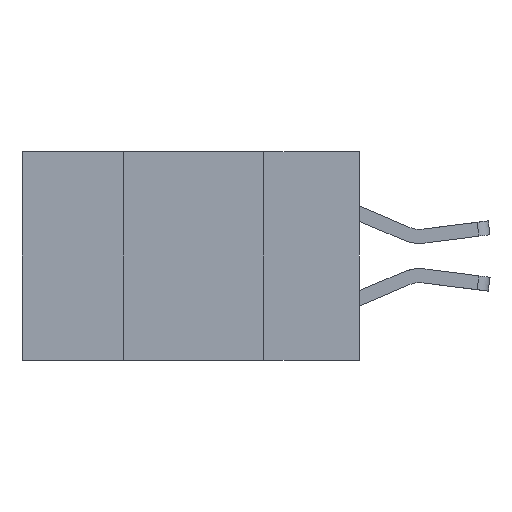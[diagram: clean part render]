
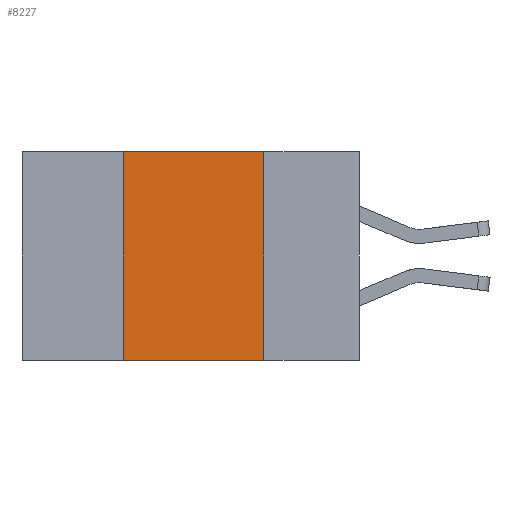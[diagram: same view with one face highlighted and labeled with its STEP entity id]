
A CAD part, left-side view. The second image highlights one B-rep face of the part: STEP entity #8227.
In plain terms, the highlighted planar face has unit normal (-1, 0, 0).
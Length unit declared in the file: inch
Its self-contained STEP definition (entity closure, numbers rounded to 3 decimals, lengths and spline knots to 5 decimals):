
#322 = LINE ( 'NONE', #11285, #13286 ) ;
#830 = LINE ( 'NONE', #6893, #8939 ) ;
#1108 = VERTEX_POINT ( 'NONE', #7104 ) ;
#1424 = DIRECTION ( 'NONE',  ( 0., 0., 1. ) ) ;
#1754 = CARTESIAN_POINT ( 'NONE',  ( 0., 0.17, 0. ) ) ;
#2039 = VECTOR ( 'NONE', #1424, 39.37008 ) ;
#2238 = PLANE ( 'NONE',  #13112 ) ;
#2888 = EDGE_CURVE ( 'NONE', #1108, #5336, #322, .T. ) ;
#3066 = EDGE_CURVE ( 'NONE', #7118, #10564, #830, .T. ) ;
#3133 = FACE_OUTER_BOUND ( 'NONE', #12243, .T. ) ;
#4411 = CARTESIAN_POINT ( 'NONE',  ( 0., 0.6, 0. ) ) ;
#4841 = EDGE_CURVE ( 'NONE', #7118, #1108, #7668, .T. ) ;
#5336 = VERTEX_POINT ( 'NONE', #9639 ) ;
#5516 = DIRECTION ( 'NONE',  ( 1., 0., 0. ) ) ;
#6893 = CARTESIAN_POINT ( 'NONE',  ( 0., 0.6, -0.37 ) ) ;
#6995 = DIRECTION ( 'NONE',  ( 0., -1., 0. ) ) ;
#7104 = CARTESIAN_POINT ( 'NONE',  ( 0., 0.42, 0. ) ) ;
#7118 = VERTEX_POINT ( 'NONE', #11430 ) ;
#7126 = DIRECTION ( 'NONE',  ( 0., 0., -1. ) ) ;
#7580 = LINE ( 'NONE', #1754, #12492 ) ;
#7668 = LINE ( 'NONE', #8759, #2039 ) ;
#8227 = ADVANCED_FACE ( 'NONE', ( #3133 ), #2238, .F. ) ;
#8576 = EDGE_CURVE ( 'NONE', #5336, #10564, #7580, .T. ) ;
#8759 = CARTESIAN_POINT ( 'NONE',  ( 0., 0.42, 0. ) ) ;
#8939 = VECTOR ( 'NONE', #6995, 39.37008 ) ;
#9639 = CARTESIAN_POINT ( 'NONE',  ( 0., 0.17, 0. ) ) ;
#10564 = VERTEX_POINT ( 'NONE', #10861 ) ;
#10861 = CARTESIAN_POINT ( 'NONE',  ( 0., 0.17, -0.37 ) ) ;
#11130 = DIRECTION ( 'NONE',  ( 0., -1., 0. ) ) ;
#11285 = CARTESIAN_POINT ( 'NONE',  ( 0., 0.6, 0. ) ) ;
#11430 = CARTESIAN_POINT ( 'NONE',  ( 0., 0.42, -0.37 ) ) ;
#12243 = EDGE_LOOP ( 'NONE', ( #12548, #12669, #12725, #12896 ) ) ;
#12454 = DIRECTION ( 'NONE',  ( 0., 0., -1. ) ) ;
#12492 = VECTOR ( 'NONE', #7126, 39.37008 ) ;
#12548 = ORIENTED_EDGE ( 'NONE', *, *, #8576, .F. ) ;
#12669 = ORIENTED_EDGE ( 'NONE', *, *, #2888, .F. ) ;
#12725 = ORIENTED_EDGE ( 'NONE', *, *, #4841, .F. ) ;
#12896 = ORIENTED_EDGE ( 'NONE', *, *, #3066, .T. ) ;
#13112 = AXIS2_PLACEMENT_3D ( 'NONE', #4411, #5516, #12454 ) ;
#13286 = VECTOR ( 'NONE', #11130, 39.37008 ) ;
